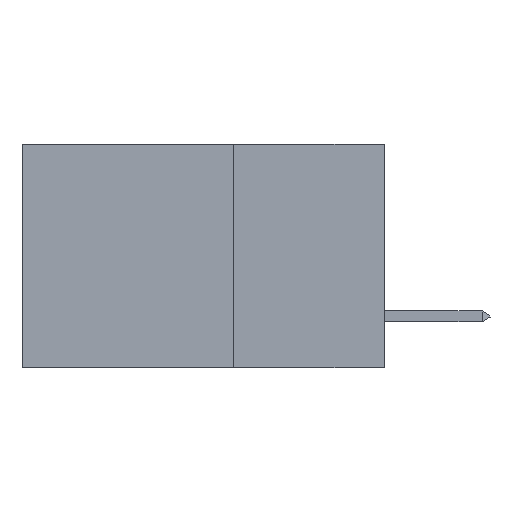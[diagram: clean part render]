
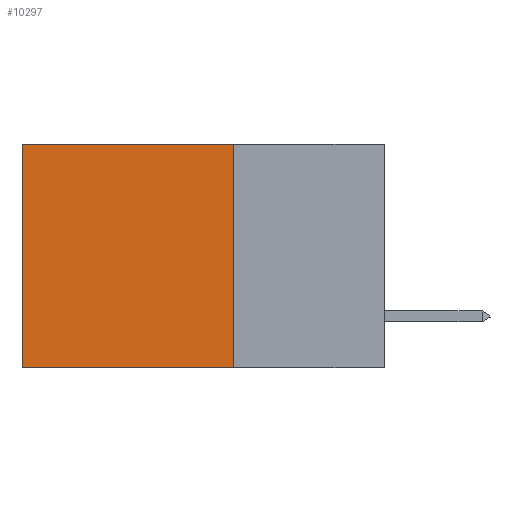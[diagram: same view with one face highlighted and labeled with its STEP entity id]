
A CAD part, left-side view. The second image highlights one B-rep face of the part: STEP entity #10297.
In plain terms, the highlighted planar face has unit normal (-1, 0, 0).
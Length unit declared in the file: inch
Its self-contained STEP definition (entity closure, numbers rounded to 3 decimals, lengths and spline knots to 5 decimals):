
#347 = ORIENTED_EDGE ( 'NONE', *, *, #13614, .F. ) ;
#942 = DIRECTION ( 'NONE',  ( 0., 0., -1. ) ) ;
#1189 = VECTOR ( 'NONE', #7488, 39.37008 ) ;
#1418 = VERTEX_POINT ( 'NONE', #9073 ) ;
#2566 = VERTEX_POINT ( 'NONE', #6990 ) ;
#4447 = LINE ( 'NONE', #10564, #6658 ) ;
#4908 = FACE_OUTER_BOUND ( 'NONE', #12880, .T. ) ;
#5266 = CARTESIAN_POINT ( 'NONE',  ( 0.2875, 0.25, 0. ) ) ;
#6651 = CARTESIAN_POINT ( 'NONE',  ( 0.2875, 0.25, 0. ) ) ;
#6658 = VECTOR ( 'NONE', #9875, 39.37008 ) ;
#6743 = DIRECTION ( 'NONE',  ( 0., 0., -1. ) ) ;
#6988 = DIRECTION ( 'NONE',  ( 0., 1., 0. ) ) ;
#6990 = CARTESIAN_POINT ( 'NONE',  ( 0.2875, 0.25, -0.37 ) ) ;
#7278 = LINE ( 'NONE', #15362, #13887 ) ;
#7488 = DIRECTION ( 'NONE',  ( 0., 0., -1. ) ) ;
#7871 = ORIENTED_EDGE ( 'NONE', *, *, #10720, .T. ) ;
#8459 = EDGE_CURVE ( 'NONE', #12560, #2566, #16539, .T. ) ;
#8666 = LINE ( 'NONE', #15830, #1189 ) ;
#9073 = CARTESIAN_POINT ( 'NONE',  ( 0.2875, 0.6, 0. ) ) ;
#9398 = VECTOR ( 'NONE', #942, 39.37008 ) ;
#9583 = EDGE_CURVE ( 'NONE', #1418, #14441, #8666, .T. ) ;
#9875 = DIRECTION ( 'NONE',  ( 0., 1., 0. ) ) ;
#10067 = ORIENTED_EDGE ( 'NONE', *, *, #9583, .T. ) ;
#10297 = ADVANCED_FACE ( 'NONE', ( #4908 ), #12219, .F. ) ;
#10564 = CARTESIAN_POINT ( 'NONE',  ( 0.2875, 0.25, -0.37 ) ) ;
#10720 = EDGE_CURVE ( 'NONE', #12560, #1418, #7278, .T. ) ;
#12219 = PLANE ( 'NONE',  #16975 ) ;
#12560 = VERTEX_POINT ( 'NONE', #12581 ) ;
#12581 = CARTESIAN_POINT ( 'NONE',  ( 0.2875, 0.25, 0. ) ) ;
#12880 = EDGE_LOOP ( 'NONE', ( #10067, #347, #15044, #7871 ) ) ;
#13614 = EDGE_CURVE ( 'NONE', #2566, #14441, #4447, .T. ) ;
#13887 = VECTOR ( 'NONE', #6988, 39.37008 ) ;
#14441 = VERTEX_POINT ( 'NONE', #15986 ) ;
#15044 = ORIENTED_EDGE ( 'NONE', *, *, #8459, .F. ) ;
#15163 = DIRECTION ( 'NONE',  ( 1., 0., 0. ) ) ;
#15362 = CARTESIAN_POINT ( 'NONE',  ( 0.2875, 0.25, 0. ) ) ;
#15830 = CARTESIAN_POINT ( 'NONE',  ( 0.2875, 0.6, 0. ) ) ;
#15986 = CARTESIAN_POINT ( 'NONE',  ( 0.2875, 0.6, -0.37 ) ) ;
#16539 = LINE ( 'NONE', #6651, #9398 ) ;
#16975 = AXIS2_PLACEMENT_3D ( 'NONE', #5266, #15163, #6743 ) ;
